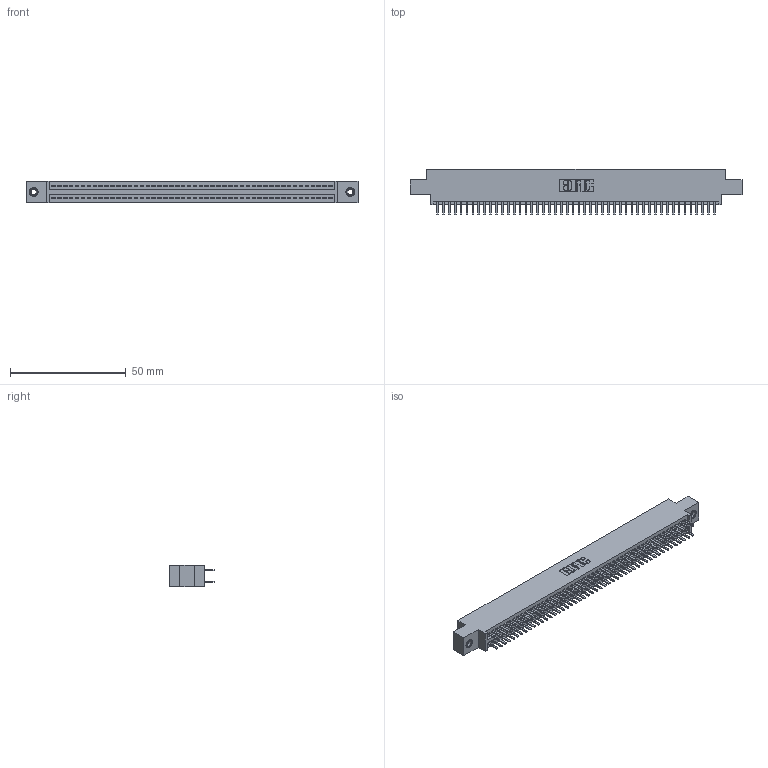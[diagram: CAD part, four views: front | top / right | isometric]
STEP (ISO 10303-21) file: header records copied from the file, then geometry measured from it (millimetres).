
FILE_DESCRIPTION (( 'STEP AP203' ), '1' );
FILE_NAME ('395-096-520-808.STEP', '2018-11-29T14:47:47', ( '' ), ( '' ), 'SwSTEP 2.0', 'SolidWorks 2016', '' );
FILE_SCHEMA (( 'CONFIG_CONTROL_DESIGN' ));
Length unit declared in the file: inch
Products named in the file (4): 345 Part_0.170 Offset - 0.156 Dia-TI; 345-292-001_345-293-120; 395-096-520-808; 345-250-001_345-250-003-102
Assembly tree (99 placements, depth 2):
  395-096-520-808
    345 Part_0.170 Offset - 0.156 Dia-TI
    345-292-001_345-293-120  x96
    345-250-001_345-250-003-102  x2
Bounding box: 143.13 x 19.68 x 9.4 mm (x, y, z)
Volume: 13797.3 mm3; surface area: 20578.1 mm2
Topology: 99 solids, 99 shells, 5374 faces, 15561 edges, 10110 vertices
Faces by surface type: plane 3476, cylinder 1882, cone 12, torus 4
Entity records: 38286 total; most frequent: CARTESIAN_POINT 6407, ORIENTED_EDGE 6322, DIRECTION 5655, EDGE_CURVE 3161, VECTOR 2813, LINE 2813, VERTEX_POINT 2100, AXIS2_PLACEMENT_3D 1421
